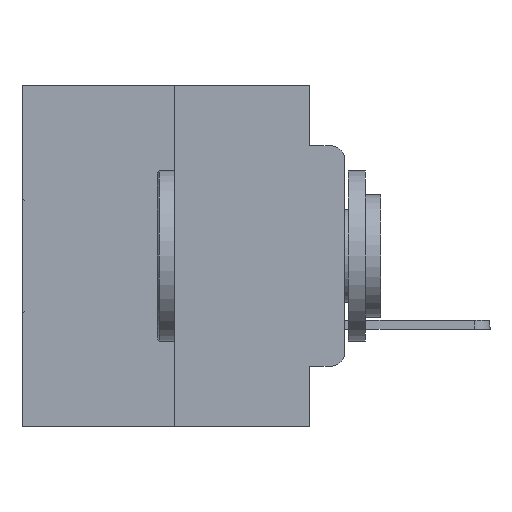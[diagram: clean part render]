
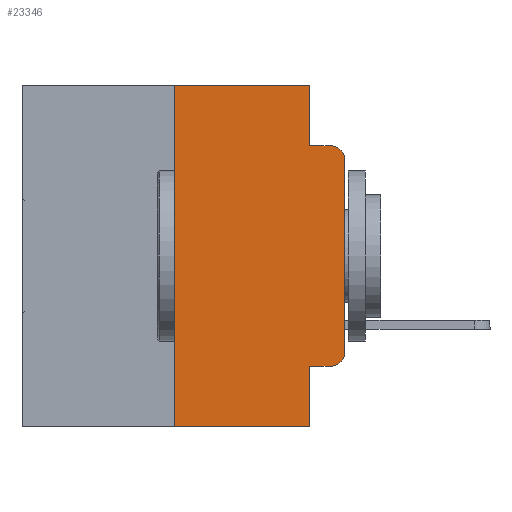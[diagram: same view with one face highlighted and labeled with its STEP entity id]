
A CAD part, left-side view. The second image highlights one B-rep face of the part: STEP entity #23346.
In plain terms, the highlighted planar face has unit normal (-1, 0, 0).
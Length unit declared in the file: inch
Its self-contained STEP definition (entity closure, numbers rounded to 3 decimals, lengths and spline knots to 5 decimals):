
#506 = LINE ( 'NONE', #14692, #15387 ) ;
#761 = VECTOR ( 'NONE', #8772, 39.37008 ) ;
#1523 = DIRECTION ( 'NONE',  ( 0., 0., -1. ) ) ;
#1531 = CARTESIAN_POINT ( 'NONE',  ( 0., 0.051, 0. ) ) ;
#1698 = CARTESIAN_POINT ( 'NONE',  ( 0., 0.473, -0.5 ) ) ;
#2274 = LINE ( 'NONE', #11901, #13006 ) ;
#2642 = VECTOR ( 'NONE', #26173, 39.37008 ) ;
#3384 = EDGE_CURVE ( 'NONE', #3474, #22233, #16686, .T. ) ;
#3433 = CARTESIAN_POINT ( 'NONE',  ( 0., 0.02, -0.1085 ) ) ;
#3474 = VERTEX_POINT ( 'NONE', #26779 ) ;
#3913 = LINE ( 'NONE', #1531, #7157 ) ;
#5126 = CIRCLE ( 'NONE', #28801, 0.02 ) ;
#5163 = CARTESIAN_POINT ( 'NONE',  ( 0., 0., 0. ) ) ;
#5576 = EDGE_CURVE ( 'NONE', #5616, #17084, #21726, .T. ) ;
#5616 = VERTEX_POINT ( 'NONE', #5956 ) ;
#5956 = CARTESIAN_POINT ( 'NONE',  ( 0., 0., -0.3915 ) ) ;
#5963 = DIRECTION ( 'NONE',  ( -1., 0., 0. ) ) ;
#6018 = VERTEX_POINT ( 'NONE', #15619 ) ;
#7157 = VECTOR ( 'NONE', #11144, 39.37008 ) ;
#7910 = VERTEX_POINT ( 'NONE', #30599 ) ;
#8201 = EDGE_CURVE ( 'NONE', #17084, #22233, #5126, .T. ) ;
#8239 = EDGE_CURVE ( 'NONE', #28900, #27857, #3913, .T. ) ;
#8475 = PLANE ( 'NONE',  #25442 ) ;
#8772 = DIRECTION ( 'NONE',  ( 0., 0., 1. ) ) ;
#8953 = ORIENTED_EDGE ( 'NONE', *, *, #30728, .T. ) ;
#9542 = DIRECTION ( 'NONE',  ( 0., -1., 0. ) ) ;
#9792 = VECTOR ( 'NONE', #21241, 39.37008 ) ;
#11144 = DIRECTION ( 'NONE',  ( 0., 0., -1. ) ) ;
#11201 = CARTESIAN_POINT ( 'NONE',  ( 0., 0., -0.1085 ) ) ;
#11618 = LINE ( 'NONE', #1698, #9792 ) ;
#11901 = CARTESIAN_POINT ( 'NONE',  ( 0., 0.473, 0. ) ) ;
#12112 = VERTEX_POINT ( 'NONE', #13114 ) ;
#12804 = DIRECTION ( 'NONE',  ( 0., 0., -1. ) ) ;
#13006 = VECTOR ( 'NONE', #9542, 39.37008 ) ;
#13046 = DIRECTION ( 'NONE',  ( 0., 0., -1. ) ) ;
#13114 = CARTESIAN_POINT ( 'NONE',  ( 0., 0.25, 0. ) ) ;
#13333 = ORIENTED_EDGE ( 'NONE', *, *, #3384, .F. ) ;
#13419 = ORIENTED_EDGE ( 'NONE', *, *, #25512, .T. ) ;
#13653 = EDGE_CURVE ( 'NONE', #28656, #5616, #16846, .T. ) ;
#13972 = CARTESIAN_POINT ( 'NONE',  ( 0., 0.02, -0.0885 ) ) ;
#14351 = VECTOR ( 'NONE', #23072, 39.37008 ) ;
#14692 = CARTESIAN_POINT ( 'NONE',  ( 0., 0.051, 0. ) ) ;
#14766 = DIRECTION ( 'NONE',  ( 0., 0., 1. ) ) ;
#15387 = VECTOR ( 'NONE', #12804, 39.37008 ) ;
#15619 = CARTESIAN_POINT ( 'NONE',  ( 0., 0.051, 0. ) ) ;
#15788 = CARTESIAN_POINT ( 'NONE',  ( 0., 0.051, -0.4115 ) ) ;
#16686 = LINE ( 'NONE', #26317, #2642 ) ;
#16846 = CIRCLE ( 'NONE', #25405, 0.02 ) ;
#17084 = VERTEX_POINT ( 'NONE', #11201 ) ;
#18072 = DIRECTION ( 'NONE',  ( -1., 0., 0. ) ) ;
#18270 = ORIENTED_EDGE ( 'NONE', *, *, #23385, .F. ) ;
#19361 = CARTESIAN_POINT ( 'NONE',  ( 0., 0.051, -0.4115 ) ) ;
#19455 = ORIENTED_EDGE ( 'NONE', *, *, #13653, .T. ) ;
#19761 = ORIENTED_EDGE ( 'NONE', *, *, #8239, .F. ) ;
#19876 = VECTOR ( 'NONE', #14766, 39.37008 ) ;
#20364 = ORIENTED_EDGE ( 'NONE', *, *, #24150, .F. ) ;
#20715 = ORIENTED_EDGE ( 'NONE', *, *, #5576, .T. ) ;
#20798 = CARTESIAN_POINT ( 'NONE',  ( 0., 0.02, -0.4115 ) ) ;
#20898 = DIRECTION ( 'NONE',  ( 0., 0., -1. ) ) ;
#21241 = DIRECTION ( 'NONE',  ( 0., -1., 0. ) ) ;
#21726 = LINE ( 'NONE', #5163, #19876 ) ;
#21792 = CARTESIAN_POINT ( 'NONE',  ( 0., 0.051, -0.5 ) ) ;
#22233 = VERTEX_POINT ( 'NONE', #13972 ) ;
#22745 = ORIENTED_EDGE ( 'NONE', *, *, #29978, .F. ) ;
#22952 = CARTESIAN_POINT ( 'NONE',  ( 0., 0.02, -0.3915 ) ) ;
#23072 = DIRECTION ( 'NONE',  ( 0., -1., 0. ) ) ;
#23346 = ADVANCED_FACE ( 'NONE', ( #28037 ), #8475, .F. ) ;
#23385 = EDGE_CURVE ( 'NONE', #7910, #12112, #28193, .T. ) ;
#24150 = EDGE_CURVE ( 'NONE', #6018, #3474, #506, .T. ) ;
#25182 = DIRECTION ( 'NONE',  ( 1., 0., 0. ) ) ;
#25405 = AXIS2_PLACEMENT_3D ( 'NONE', #22952, #18072, #20898 ) ;
#25442 = AXIS2_PLACEMENT_3D ( 'NONE', #30237, #25182, #1523 ) ;
#25512 = EDGE_CURVE ( 'NONE', #28900, #28656, #27492, .T. ) ;
#26173 = DIRECTION ( 'NONE',  ( 0., -1., 0. ) ) ;
#26317 = CARTESIAN_POINT ( 'NONE',  ( 0., 0.051, -0.0885 ) ) ;
#26779 = CARTESIAN_POINT ( 'NONE',  ( 0., 0.051, -0.0885 ) ) ;
#27492 = LINE ( 'NONE', #15788, #14351 ) ;
#27607 = EDGE_LOOP ( 'NONE', ( #20715, #30695, #13333, #20364, #22745, #18270, #8953, #19761, #13419, #19455 ) ) ;
#27857 = VERTEX_POINT ( 'NONE', #21792 ) ;
#27871 = CARTESIAN_POINT ( 'NONE',  ( 0., 0.25, 0. ) ) ;
#28037 = FACE_OUTER_BOUND ( 'NONE', #27607, .T. ) ;
#28193 = LINE ( 'NONE', #27871, #761 ) ;
#28656 = VERTEX_POINT ( 'NONE', #20798 ) ;
#28801 = AXIS2_PLACEMENT_3D ( 'NONE', #3433, #5963, #13046 ) ;
#28900 = VERTEX_POINT ( 'NONE', #19361 ) ;
#29978 = EDGE_CURVE ( 'NONE', #12112, #6018, #2274, .T. ) ;
#30237 = CARTESIAN_POINT ( 'NONE',  ( 0., 0.473, 0. ) ) ;
#30599 = CARTESIAN_POINT ( 'NONE',  ( 0., 0.25, -0.5 ) ) ;
#30695 = ORIENTED_EDGE ( 'NONE', *, *, #8201, .T. ) ;
#30728 = EDGE_CURVE ( 'NONE', #7910, #27857, #11618, .T. ) ;
